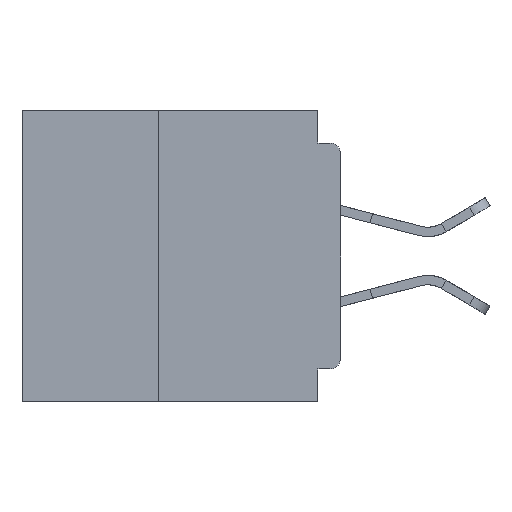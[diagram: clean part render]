
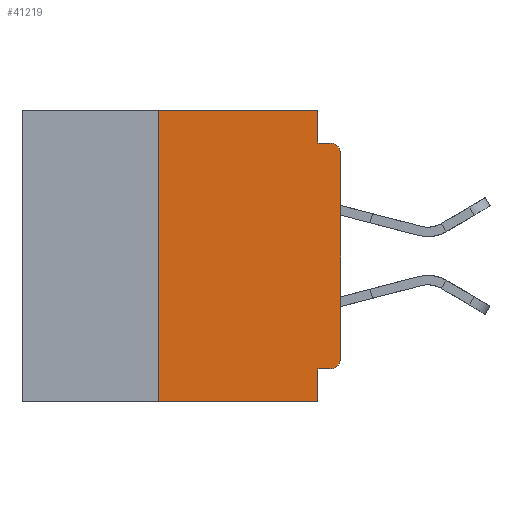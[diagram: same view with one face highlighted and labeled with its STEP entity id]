
A CAD part, left-side view. The second image highlights one B-rep face of the part: STEP entity #41219.
In plain terms, the highlighted planar face has unit normal (-1, 0, 0).
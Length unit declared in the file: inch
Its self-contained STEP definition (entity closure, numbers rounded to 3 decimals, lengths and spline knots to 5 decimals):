
#127 = VERTEX_POINT ( 'NONE', #25367 ) ;
#264 = CIRCLE ( 'NONE', #28550, 0.015 ) ;
#1015 = EDGE_CURVE ( 'NONE', #38437, #127, #24256, .T. ) ;
#1992 = EDGE_CURVE ( 'NONE', #10736, #20419, #13562, .T. ) ;
#2149 = DIRECTION ( 'NONE',  ( 0., 0., -1. ) ) ;
#3025 = VERTEX_POINT ( 'NONE', #36948 ) ;
#3555 = ORIENTED_EDGE ( 'NONE', *, *, #40143, .T. ) ;
#4008 = VECTOR ( 'NONE', #34593, 39.37008 ) ;
#4047 = CARTESIAN_POINT ( 'NONE',  ( 0., 0., 0. ) ) ;
#4062 = CARTESIAN_POINT ( 'NONE',  ( 0., 0.25, -0.4 ) ) ;
#4998 = DIRECTION ( 'NONE',  ( 0., 0., -1. ) ) ;
#5315 = LINE ( 'NONE', #7898, #28926 ) ;
#5759 = VECTOR ( 'NONE', #39406, 39.37008 ) ;
#6471 = CARTESIAN_POINT ( 'NONE',  ( 0., 0.031, 0. ) ) ;
#6809 = CARTESIAN_POINT ( 'NONE',  ( 0., 0.031, -0.045 ) ) ;
#7898 = CARTESIAN_POINT ( 'NONE',  ( 0., 0.437, 0. ) ) ;
#8200 = CARTESIAN_POINT ( 'NONE',  ( 0., 0.437, -0.4 ) ) ;
#10290 = CARTESIAN_POINT ( 'NONE',  ( 0., 0.015, -0.355 ) ) ;
#10402 = DIRECTION ( 'NONE',  ( 0., -1., 0. ) ) ;
#10579 = ORIENTED_EDGE ( 'NONE', *, *, #11957, .F. ) ;
#10618 = CARTESIAN_POINT ( 'NONE',  ( 0., 0., -0.06 ) ) ;
#10736 = VERTEX_POINT ( 'NONE', #10290 ) ;
#11148 = DIRECTION ( 'NONE',  ( 0., -1., 0. ) ) ;
#11463 = ORIENTED_EDGE ( 'NONE', *, *, #1992, .F. ) ;
#11529 = LINE ( 'NONE', #16767, #17088 ) ;
#11793 = CARTESIAN_POINT ( 'NONE',  ( 0., 0.031, -0.355 ) ) ;
#11957 = EDGE_CURVE ( 'NONE', #38437, #31810, #14770, .T. ) ;
#12226 = LINE ( 'NONE', #26076, #36832 ) ;
#13418 = CARTESIAN_POINT ( 'NONE',  ( 0., 0., -0.355 ) ) ;
#13562 = LINE ( 'NONE', #13418, #4008 ) ;
#14056 = VERTEX_POINT ( 'NONE', #31521 ) ;
#14322 = LINE ( 'NONE', #4047, #5759 ) ;
#14444 = ORIENTED_EDGE ( 'NONE', *, *, #1015, .T. ) ;
#14770 = LINE ( 'NONE', #16396, #30802 ) ;
#14935 = EDGE_CURVE ( 'NONE', #40886, #14056, #11529, .T. ) ;
#14947 = PLANE ( 'NONE',  #23230 ) ;
#14977 = DIRECTION ( 'NONE',  ( -1., 0., 0. ) ) ;
#16396 = CARTESIAN_POINT ( 'NONE',  ( 0., 0.25, -0.4 ) ) ;
#16767 = CARTESIAN_POINT ( 'NONE',  ( 0., 0., -0.045 ) ) ;
#17088 = VECTOR ( 'NONE', #10402, 39.37008 ) ;
#17286 = EDGE_CURVE ( 'NONE', #31810, #38265, #5315, .T. ) ;
#17819 = DIRECTION ( 'NONE',  ( 0., 0., -1. ) ) ;
#18183 = CARTESIAN_POINT ( 'NONE',  ( 0., 0.437, 0. ) ) ;
#19018 = VERTEX_POINT ( 'NONE', #10618 ) ;
#19189 = EDGE_CURVE ( 'NONE', #38265, #40886, #40338, .T. ) ;
#19269 = DIRECTION ( 'NONE',  ( -1., 0., 0. ) ) ;
#20419 = VERTEX_POINT ( 'NONE', #11793 ) ;
#21445 = DIRECTION ( 'NONE',  ( 1., 0., 0. ) ) ;
#21811 = ORIENTED_EDGE ( 'NONE', *, *, #17286, .F. ) ;
#22442 = DIRECTION ( 'NONE',  ( 0., -1., 0. ) ) ;
#22854 = DIRECTION ( 'NONE',  ( 0., 0., -1. ) ) ;
#22894 = DIRECTION ( 'NONE',  ( 0., 0., 1. ) ) ;
#23230 = AXIS2_PLACEMENT_3D ( 'NONE', #18183, #21445, #2149 ) ;
#23595 = ORIENTED_EDGE ( 'NONE', *, *, #33679, .T. ) ;
#24147 = CIRCLE ( 'NONE', #35735, 0.015 ) ;
#24256 = LINE ( 'NONE', #8200, #40231 ) ;
#25367 = CARTESIAN_POINT ( 'NONE',  ( 0., 0.031, -0.4 ) ) ;
#25878 = ORIENTED_EDGE ( 'NONE', *, *, #37359, .T. ) ;
#26076 = CARTESIAN_POINT ( 'NONE',  ( 0., 0.031, -0.4 ) ) ;
#26966 = EDGE_CURVE ( 'NONE', #20419, #127, #12226, .T. ) ;
#28164 = ORIENTED_EDGE ( 'NONE', *, *, #19189, .F. ) ;
#28165 = ORIENTED_EDGE ( 'NONE', *, *, #26966, .F. ) ;
#28550 = AXIS2_PLACEMENT_3D ( 'NONE', #38464, #19269, #17819 ) ;
#28591 = CARTESIAN_POINT ( 'NONE',  ( 0., 0.25, 0. ) ) ;
#28926 = VECTOR ( 'NONE', #11148, 39.37008 ) ;
#30547 = EDGE_LOOP ( 'NONE', ( #23595, #25878, #38888, #28164, #21811, #10579, #14444, #28165, #11463, #3555 ) ) ;
#30802 = VECTOR ( 'NONE', #22894, 39.37008 ) ;
#30807 = VECTOR ( 'NONE', #4998, 39.37008 ) ;
#31521 = CARTESIAN_POINT ( 'NONE',  ( 0., 0.015, -0.045 ) ) ;
#31810 = VERTEX_POINT ( 'NONE', #28591 ) ;
#33679 = EDGE_CURVE ( 'NONE', #3025, #19018, #14322, .T. ) ;
#33873 = CARTESIAN_POINT ( 'NONE',  ( 0., 0.031, 0. ) ) ;
#34155 = CARTESIAN_POINT ( 'NONE',  ( 0., 0.015, -0.06 ) ) ;
#34593 = DIRECTION ( 'NONE',  ( 0., 1., 0. ) ) ;
#35735 = AXIS2_PLACEMENT_3D ( 'NONE', #34155, #14977, #37427 ) ;
#36832 = VECTOR ( 'NONE', #22854, 39.37008 ) ;
#36948 = CARTESIAN_POINT ( 'NONE',  ( 0., 0., -0.34 ) ) ;
#37359 = EDGE_CURVE ( 'NONE', #19018, #14056, #24147, .T. ) ;
#37427 = DIRECTION ( 'NONE',  ( 0., 0., -1. ) ) ;
#38265 = VERTEX_POINT ( 'NONE', #6471 ) ;
#38437 = VERTEX_POINT ( 'NONE', #4062 ) ;
#38464 = CARTESIAN_POINT ( 'NONE',  ( 0., 0.015, -0.34 ) ) ;
#38888 = ORIENTED_EDGE ( 'NONE', *, *, #14935, .F. ) ;
#39406 = DIRECTION ( 'NONE',  ( 0., 0., 1. ) ) ;
#40143 = EDGE_CURVE ( 'NONE', #10736, #3025, #264, .T. ) ;
#40231 = VECTOR ( 'NONE', #22442, 39.37008 ) ;
#40338 = LINE ( 'NONE', #33873, #30807 ) ;
#40886 = VERTEX_POINT ( 'NONE', #6809 ) ;
#41219 = ADVANCED_FACE ( 'NONE', ( #41358 ), #14947, .F. ) ;
#41358 = FACE_OUTER_BOUND ( 'NONE', #30547, .T. ) ;
